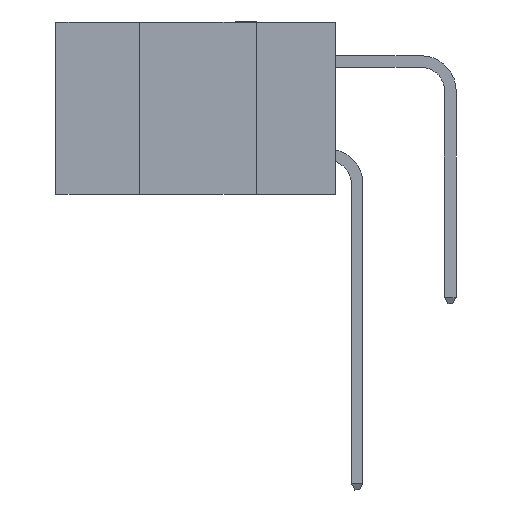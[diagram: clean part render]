
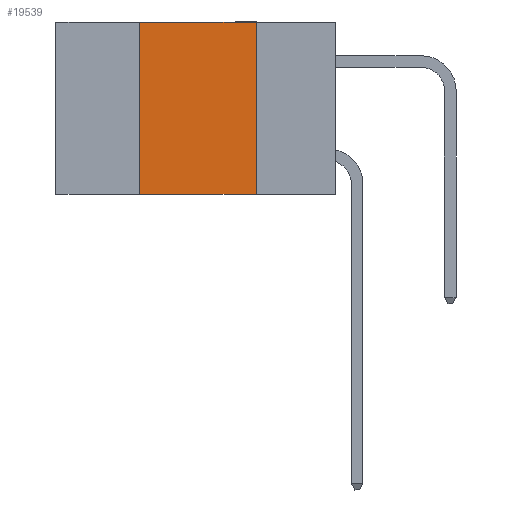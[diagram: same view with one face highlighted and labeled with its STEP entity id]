
A CAD part, left-side view. The second image highlights one B-rep face of the part: STEP entity #19539.
In plain terms, the highlighted planar face has unit normal (-1, 0, 0).
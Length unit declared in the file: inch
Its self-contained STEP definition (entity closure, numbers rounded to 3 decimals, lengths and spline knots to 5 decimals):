
#721 = FACE_OUTER_BOUND ( 'NONE', #11051, .T. ) ;
#941 = DIRECTION ( 'NONE',  ( 0., 0., -1. ) ) ;
#1839 = VERTEX_POINT ( 'NONE', #9577 ) ;
#2105 = EDGE_CURVE ( 'NONE', #9267, #15053, #8192, .T. ) ;
#2372 = CARTESIAN_POINT ( 'NONE',  ( 0., 0.42, -0.37 ) ) ;
#2467 = CARTESIAN_POINT ( 'NONE',  ( 0., 0.42, 0. ) ) ;
#2832 = AXIS2_PLACEMENT_3D ( 'NONE', #6003, #17923, #9019 ) ;
#3968 = EDGE_CURVE ( 'NONE', #18173, #15053, #10224, .T. ) ;
#4226 = LINE ( 'NONE', #2467, #11823 ) ;
#5479 = DIRECTION ( 'NONE',  ( 0., -1., 0. ) ) ;
#5689 = CARTESIAN_POINT ( 'NONE',  ( 0., 0.17, 0. ) ) ;
#5701 = EDGE_CURVE ( 'NONE', #18173, #1839, #4226, .T. ) ;
#5801 = CARTESIAN_POINT ( 'NONE',  ( 0., 0.6, 0. ) ) ;
#6003 = CARTESIAN_POINT ( 'NONE',  ( 0., 0.6, 0. ) ) ;
#6235 = VECTOR ( 'NONE', #5479, 39.37008 ) ;
#6946 = CARTESIAN_POINT ( 'NONE',  ( 0., 0.17, 0. ) ) ;
#7516 = PLANE ( 'NONE',  #2832 ) ;
#8192 = LINE ( 'NONE', #5689, #19113 ) ;
#9019 = DIRECTION ( 'NONE',  ( 0., 0., -1. ) ) ;
#9267 = VERTEX_POINT ( 'NONE', #6946 ) ;
#9577 = CARTESIAN_POINT ( 'NONE',  ( 0., 0.42, 0. ) ) ;
#9966 = LINE ( 'NONE', #5801, #13925 ) ;
#10224 = LINE ( 'NONE', #15952, #6235 ) ;
#10739 = ORIENTED_EDGE ( 'NONE', *, *, #2105, .F. ) ;
#11051 = EDGE_LOOP ( 'NONE', ( #10739, #14706, #15170, #19077 ) ) ;
#11823 = VECTOR ( 'NONE', #14661, 39.37008 ) ;
#13925 = VECTOR ( 'NONE', #16255, 39.37008 ) ;
#14661 = DIRECTION ( 'NONE',  ( 0., 0., 1. ) ) ;
#14706 = ORIENTED_EDGE ( 'NONE', *, *, #19446, .F. ) ;
#15053 = VERTEX_POINT ( 'NONE', #16577 ) ;
#15170 = ORIENTED_EDGE ( 'NONE', *, *, #5701, .F. ) ;
#15952 = CARTESIAN_POINT ( 'NONE',  ( 0., 0.6, -0.37 ) ) ;
#16255 = DIRECTION ( 'NONE',  ( 0., -1., 0. ) ) ;
#16577 = CARTESIAN_POINT ( 'NONE',  ( 0., 0.17, -0.37 ) ) ;
#17923 = DIRECTION ( 'NONE',  ( 1., 0., 0. ) ) ;
#18173 = VERTEX_POINT ( 'NONE', #2372 ) ;
#19077 = ORIENTED_EDGE ( 'NONE', *, *, #3968, .T. ) ;
#19113 = VECTOR ( 'NONE', #941, 39.37008 ) ;
#19446 = EDGE_CURVE ( 'NONE', #1839, #9267, #9966, .T. ) ;
#19539 = ADVANCED_FACE ( 'NONE', ( #721 ), #7516, .F. ) ;
